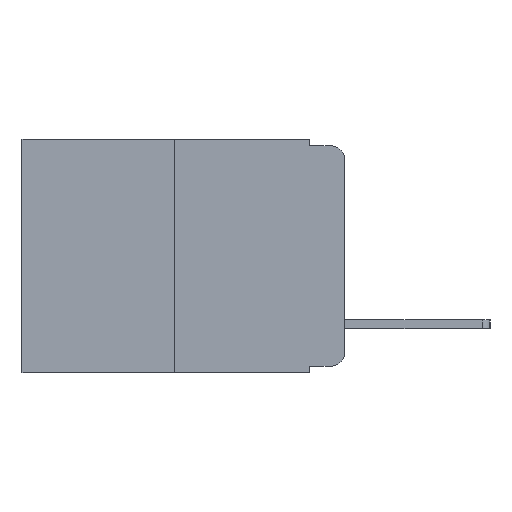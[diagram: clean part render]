
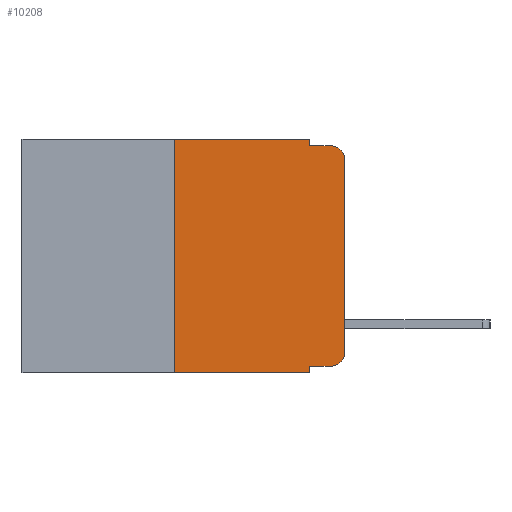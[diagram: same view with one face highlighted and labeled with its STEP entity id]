
A CAD part, left-side view. The second image highlights one B-rep face of the part: STEP entity #10208.
In plain terms, the highlighted planar face has unit normal (-1, 0, 0).
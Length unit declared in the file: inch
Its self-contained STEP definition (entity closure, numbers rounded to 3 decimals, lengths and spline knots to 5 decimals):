
#120 = CIRCLE ( 'NONE', #4391, 0.02 ) ;
#127 = DIRECTION ( 'NONE',  ( 1., 0., 0. ) ) ;
#628 = CARTESIAN_POINT ( 'NONE',  ( 0., 0.473, 0. ) ) ;
#703 = CARTESIAN_POINT ( 'NONE',  ( 0., 0.051, -0.01 ) ) ;
#742 = ORIENTED_EDGE ( 'NONE', *, *, #9243, .F. ) ;
#1102 = ORIENTED_EDGE ( 'NONE', *, *, #6919, .T. ) ;
#1216 = VERTEX_POINT ( 'NONE', #10366 ) ;
#1281 = DIRECTION ( 'NONE',  ( 0., 0., 1. ) ) ;
#1550 = EDGE_CURVE ( 'NONE', #2998, #6394, #4974, .T. ) ;
#1655 = DIRECTION ( 'NONE',  ( -1., 0., 0. ) ) ;
#1713 = CARTESIAN_POINT ( 'NONE',  ( 0., 0.051, -0.343 ) ) ;
#1992 = CARTESIAN_POINT ( 'NONE',  ( 0., 0.473, -0.343 ) ) ;
#2112 = DIRECTION ( 'NONE',  ( 0., 0., -1. ) ) ;
#2195 = CARTESIAN_POINT ( 'NONE',  ( 0., 0.051, 0. ) ) ;
#2255 = DIRECTION ( 'NONE',  ( 0., -1., 0. ) ) ;
#2286 = VERTEX_POINT ( 'NONE', #4568 ) ;
#2328 = VERTEX_POINT ( 'NONE', #6050 ) ;
#2687 = EDGE_LOOP ( 'NONE', ( #6901, #9706, #7620, #5334, #742, #5706, #8687, #5277, #3546, #1102 ) ) ;
#2772 = LINE ( 'NONE', #6756, #7671 ) ;
#2799 = VERTEX_POINT ( 'NONE', #4756 ) ;
#2834 = CARTESIAN_POINT ( 'NONE',  ( 0., 0.051, -0.333 ) ) ;
#2847 = DIRECTION ( 'NONE',  ( 0., 0., -1. ) ) ;
#2907 = EDGE_CURVE ( 'NONE', #9891, #6725, #8722, .T. ) ;
#2928 = EDGE_CURVE ( 'NONE', #9891, #2286, #6030, .T. ) ;
#2998 = VERTEX_POINT ( 'NONE', #703 ) ;
#3068 = AXIS2_PLACEMENT_3D ( 'NONE', #7146, #1655, #8045 ) ;
#3546 = ORIENTED_EDGE ( 'NONE', *, *, #2928, .T. ) ;
#3755 = EDGE_CURVE ( 'NONE', #1216, #6394, #120, .T. ) ;
#3826 = EDGE_CURVE ( 'NONE', #8739, #2998, #6859, .T. ) ;
#3851 = DIRECTION ( 'NONE',  ( 0., 0., 1. ) ) ;
#4018 = LINE ( 'NONE', #628, #10381 ) ;
#4391 = AXIS2_PLACEMENT_3D ( 'NONE', #9393, #9376, #7791 ) ;
#4568 = CARTESIAN_POINT ( 'NONE',  ( 0., 0.02, -0.333 ) ) ;
#4756 = CARTESIAN_POINT ( 'NONE',  ( 0., 0.25, 0. ) ) ;
#4974 = LINE ( 'NONE', #8746, #10064 ) ;
#5180 = CARTESIAN_POINT ( 'NONE',  ( 0., 0.051, -0.333 ) ) ;
#5193 = CARTESIAN_POINT ( 'NONE',  ( 0., 0.25, -0.343 ) ) ;
#5224 = EDGE_CURVE ( 'NONE', #8732, #2799, #10444, .T. ) ;
#5277 = ORIENTED_EDGE ( 'NONE', *, *, #2907, .F. ) ;
#5334 = ORIENTED_EDGE ( 'NONE', *, *, #3826, .F. ) ;
#5630 = CARTESIAN_POINT ( 'NONE',  ( 0., 0.473, 0. ) ) ;
#5706 = ORIENTED_EDGE ( 'NONE', *, *, #5224, .F. ) ;
#5743 = VECTOR ( 'NONE', #2255, 39.37008 ) ;
#5842 = FACE_OUTER_BOUND ( 'NONE', #2687, .T. ) ;
#5919 = CARTESIAN_POINT ( 'NONE',  ( 0., 0.051, 0. ) ) ;
#6030 = LINE ( 'NONE', #2834, #5743 ) ;
#6050 = CARTESIAN_POINT ( 'NONE',  ( 0., 0., -0.313 ) ) ;
#6376 = CARTESIAN_POINT ( 'NONE',  ( 0., 0.25, 0. ) ) ;
#6394 = VERTEX_POINT ( 'NONE', #7683 ) ;
#6485 = PLANE ( 'NONE',  #9152 ) ;
#6526 = DIRECTION ( 'NONE',  ( 0., 0., -1. ) ) ;
#6559 = VECTOR ( 'NONE', #2847, 39.37008 ) ;
#6609 = VECTOR ( 'NONE', #8380, 39.37008 ) ;
#6725 = VERTEX_POINT ( 'NONE', #1713 ) ;
#6756 = CARTESIAN_POINT ( 'NONE',  ( 0., 0., 0. ) ) ;
#6859 = LINE ( 'NONE', #5919, #6559 ) ;
#6901 = ORIENTED_EDGE ( 'NONE', *, *, #11003, .T. ) ;
#6913 = LINE ( 'NONE', #1992, #6609 ) ;
#6919 = EDGE_CURVE ( 'NONE', #2286, #2328, #11242, .T. ) ;
#7146 = CARTESIAN_POINT ( 'NONE',  ( 0., 0.02, -0.313 ) ) ;
#7620 = ORIENTED_EDGE ( 'NONE', *, *, #1550, .F. ) ;
#7671 = VECTOR ( 'NONE', #1281, 39.37008 ) ;
#7683 = CARTESIAN_POINT ( 'NONE',  ( 0., 0.02, -0.01 ) ) ;
#7791 = DIRECTION ( 'NONE',  ( 0., 0., -1. ) ) ;
#7934 = DIRECTION ( 'NONE',  ( 0., -1., 0. ) ) ;
#7981 = CARTESIAN_POINT ( 'NONE',  ( 0., 0.051, 0. ) ) ;
#8045 = DIRECTION ( 'NONE',  ( 0., 0., -1. ) ) ;
#8093 = VECTOR ( 'NONE', #3851, 39.37008 ) ;
#8380 = DIRECTION ( 'NONE',  ( 0., -1., 0. ) ) ;
#8434 = VECTOR ( 'NONE', #2112, 39.37008 ) ;
#8687 = ORIENTED_EDGE ( 'NONE', *, *, #8902, .T. ) ;
#8722 = LINE ( 'NONE', #2195, #8434 ) ;
#8732 = VERTEX_POINT ( 'NONE', #5193 ) ;
#8739 = VERTEX_POINT ( 'NONE', #7981 ) ;
#8746 = CARTESIAN_POINT ( 'NONE',  ( 0., 0.051, -0.01 ) ) ;
#8902 = EDGE_CURVE ( 'NONE', #8732, #6725, #6913, .T. ) ;
#9152 = AXIS2_PLACEMENT_3D ( 'NONE', #5630, #127, #6526 ) ;
#9243 = EDGE_CURVE ( 'NONE', #2799, #8739, #4018, .T. ) ;
#9376 = DIRECTION ( 'NONE',  ( -1., 0., 0. ) ) ;
#9393 = CARTESIAN_POINT ( 'NONE',  ( 0., 0.02, -0.03 ) ) ;
#9706 = ORIENTED_EDGE ( 'NONE', *, *, #3755, .T. ) ;
#9866 = DIRECTION ( 'NONE',  ( 0., -1., 0. ) ) ;
#9891 = VERTEX_POINT ( 'NONE', #5180 ) ;
#10064 = VECTOR ( 'NONE', #9866, 39.37008 ) ;
#10208 = ADVANCED_FACE ( 'NONE', ( #5842 ), #6485, .F. ) ;
#10366 = CARTESIAN_POINT ( 'NONE',  ( 0., 0., -0.03 ) ) ;
#10381 = VECTOR ( 'NONE', #7934, 39.37008 ) ;
#10444 = LINE ( 'NONE', #6376, #8093 ) ;
#11003 = EDGE_CURVE ( 'NONE', #2328, #1216, #2772, .T. ) ;
#11242 = CIRCLE ( 'NONE', #3068, 0.02 ) ;
